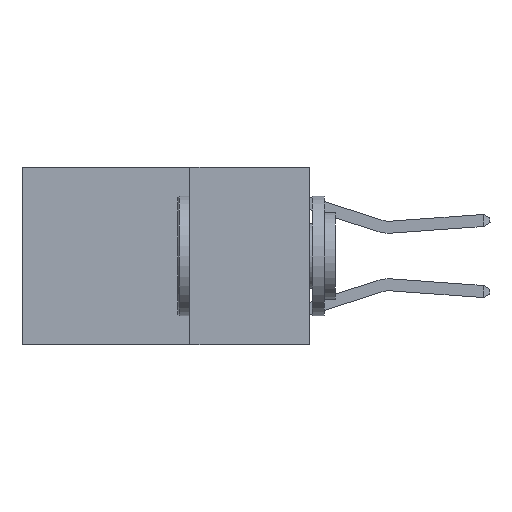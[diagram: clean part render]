
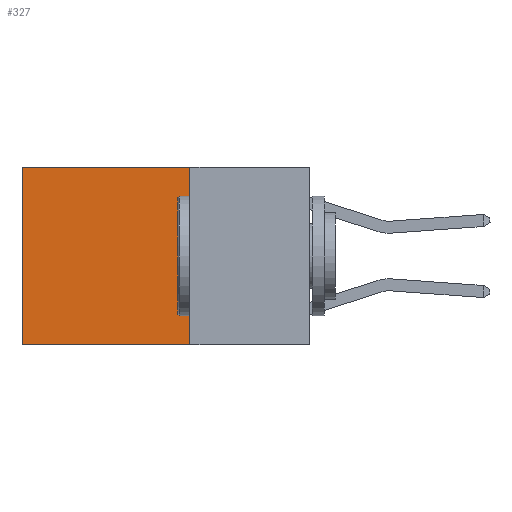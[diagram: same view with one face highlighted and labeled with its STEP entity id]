
A CAD part, left-side view. The second image highlights one B-rep face of the part: STEP entity #327.
In plain terms, the highlighted planar face has unit normal (-1, 0, 0).
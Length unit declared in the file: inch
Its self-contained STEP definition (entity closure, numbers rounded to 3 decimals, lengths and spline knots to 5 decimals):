
#234 = ORIENTED_EDGE ( 'NONE', *, *, #8765, .F. ) ;
#327 = ADVANCED_FACE ( 'NONE', ( #2697 ), #6227, .F. ) ;
#622 = LINE ( 'NONE', #710, #3151 ) ;
#710 = CARTESIAN_POINT ( 'NONE',  ( 0.2625, 0.6, 0. ) ) ;
#760 = DIRECTION ( 'NONE',  ( 0., 0., -1. ) ) ;
#948 = DIRECTION ( 'NONE',  ( 0., 1., 0. ) ) ;
#1074 = EDGE_CURVE ( 'NONE', #5093, #1241, #6077, .T. ) ;
#1091 = DIRECTION ( 'NONE',  ( 0., 0., -1. ) ) ;
#1241 = VERTEX_POINT ( 'NONE', #8677 ) ;
#1323 = CARTESIAN_POINT ( 'NONE',  ( 0.2625, 0.25, 0. ) ) ;
#1395 = CARTESIAN_POINT ( 'NONE',  ( 0.2625, 0.6, 0. ) ) ;
#1787 = DIRECTION ( 'NONE',  ( 0., 1., 0. ) ) ;
#2399 = VECTOR ( 'NONE', #1787, 39.37008 ) ;
#2412 = EDGE_LOOP ( 'NONE', ( #8204, #234, #11123, #3491 ) ) ;
#2468 = VECTOR ( 'NONE', #948, 39.37008 ) ;
#2697 = FACE_OUTER_BOUND ( 'NONE', #2412, .T. ) ;
#3151 = VECTOR ( 'NONE', #760, 39.37008 ) ;
#3426 = VECTOR ( 'NONE', #1091, 39.37008 ) ;
#3491 = ORIENTED_EDGE ( 'NONE', *, *, #4166, .T. ) ;
#4166 = EDGE_CURVE ( 'NONE', #5093, #9927, #5080, .T. ) ;
#4969 = CARTESIAN_POINT ( 'NONE',  ( 0.2625, 0.25, 0. ) ) ;
#5080 = LINE ( 'NONE', #7854, #2399 ) ;
#5093 = VERTEX_POINT ( 'NONE', #4969 ) ;
#5868 = EDGE_CURVE ( 'NONE', #9927, #6843, #622, .T. ) ;
#5947 = DIRECTION ( 'NONE',  ( 0., 0., -1. ) ) ;
#6077 = LINE ( 'NONE', #1323, #3426 ) ;
#6183 = DIRECTION ( 'NONE',  ( 1., 0., 0. ) ) ;
#6227 = PLANE ( 'NONE',  #11487 ) ;
#6261 = CARTESIAN_POINT ( 'NONE',  ( 0.2625, 0.25, 0. ) ) ;
#6843 = VERTEX_POINT ( 'NONE', #6992 ) ;
#6992 = CARTESIAN_POINT ( 'NONE',  ( 0.2625, 0.6, -0.37 ) ) ;
#7077 = CARTESIAN_POINT ( 'NONE',  ( 0.2625, 0.25, -0.37 ) ) ;
#7854 = CARTESIAN_POINT ( 'NONE',  ( 0.2625, 0.25, 0. ) ) ;
#8204 = ORIENTED_EDGE ( 'NONE', *, *, #5868, .T. ) ;
#8677 = CARTESIAN_POINT ( 'NONE',  ( 0.2625, 0.25, -0.37 ) ) ;
#8765 = EDGE_CURVE ( 'NONE', #1241, #6843, #12693, .T. ) ;
#9927 = VERTEX_POINT ( 'NONE', #1395 ) ;
#11123 = ORIENTED_EDGE ( 'NONE', *, *, #1074, .F. ) ;
#11487 = AXIS2_PLACEMENT_3D ( 'NONE', #6261, #6183, #5947 ) ;
#12693 = LINE ( 'NONE', #7077, #2468 ) ;
